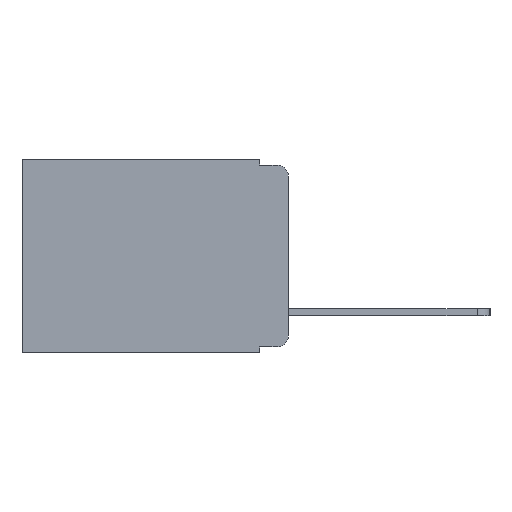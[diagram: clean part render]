
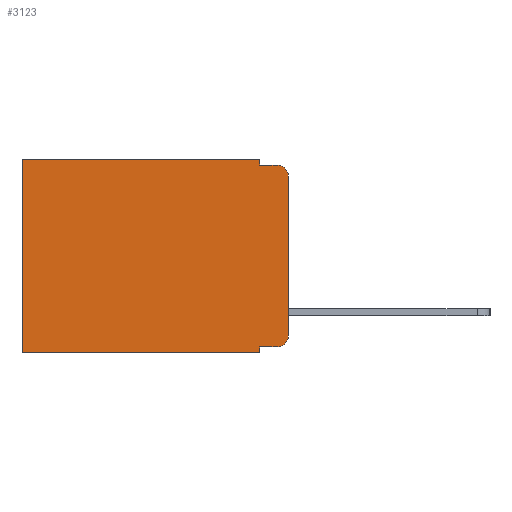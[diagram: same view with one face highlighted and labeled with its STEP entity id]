
A CAD part, left-side view. The second image highlights one B-rep face of the part: STEP entity #3123.
In plain terms, the highlighted planar face has unit normal (-1, 0, 0).
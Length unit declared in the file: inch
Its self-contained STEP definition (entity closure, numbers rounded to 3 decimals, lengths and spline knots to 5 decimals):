
#327 = ORIENTED_EDGE ( 'NONE', *, *, #18414, .F. ) ;
#622 = CARTESIAN_POINT ( 'NONE',  ( 0.298, 0., 0. ) ) ;
#1274 = CARTESIAN_POINT ( 'NONE',  ( 0.298, 0.473, 0. ) ) ;
#1833 = VERTEX_POINT ( 'NONE', #5368 ) ;
#2019 = ORIENTED_EDGE ( 'NONE', *, *, #11869, .T. ) ;
#2214 = VERTEX_POINT ( 'NONE', #1274 ) ;
#2249 = EDGE_CURVE ( 'NONE', #18084, #2214, #5671, .T. ) ;
#2390 = CARTESIAN_POINT ( 'NONE',  ( 0.298, 0.051, 0. ) ) ;
#2619 = VERTEX_POINT ( 'NONE', #6389 ) ;
#2701 = ORIENTED_EDGE ( 'NONE', *, *, #6005, .F. ) ;
#2780 = ORIENTED_EDGE ( 'NONE', *, *, #13232, .F. ) ;
#2804 = ORIENTED_EDGE ( 'NONE', *, *, #17581, .F. ) ;
#2856 = VERTEX_POINT ( 'NONE', #7756 ) ;
#2863 = DIRECTION ( 'NONE',  ( 0., 0., -1. ) ) ;
#2877 = CARTESIAN_POINT ( 'NONE',  ( 0.298, 0.051, -0.01 ) ) ;
#2908 = EDGE_CURVE ( 'NONE', #12253, #18066, #9824, .T. ) ;
#2993 = DIRECTION ( 'NONE',  ( 0., 0., -1. ) ) ;
#3123 = ADVANCED_FACE ( 'NONE', ( #16680 ), #18057, .F. ) ;
#3352 = VECTOR ( 'NONE', #12603, 39.37008 ) ;
#3385 = CARTESIAN_POINT ( 'NONE',  ( 0.298, 0., -0.313 ) ) ;
#3512 = CARTESIAN_POINT ( 'NONE',  ( 0.298, 0.02, -0.333 ) ) ;
#3734 = VECTOR ( 'NONE', #4436, 39.37008 ) ;
#3966 = DIRECTION ( 'NONE',  ( -1., 0., 0. ) ) ;
#3967 = DIRECTION ( 'NONE',  ( 0., 0., -1. ) ) ;
#4007 = CIRCLE ( 'NONE', #10460, 0.02 ) ;
#4109 = VERTEX_POINT ( 'NONE', #3385 ) ;
#4436 = DIRECTION ( 'NONE',  ( 0., -1., 0. ) ) ;
#4811 = CARTESIAN_POINT ( 'NONE',  ( 0.298, 0., -0.03 ) ) ;
#5027 = ORIENTED_EDGE ( 'NONE', *, *, #2908, .T. ) ;
#5180 = ORIENTED_EDGE ( 'NONE', *, *, #15065, .F. ) ;
#5368 = CARTESIAN_POINT ( 'NONE',  ( 0.298, 0.051, -0.01 ) ) ;
#5398 = CARTESIAN_POINT ( 'NONE',  ( 0.298, 0.051, 0. ) ) ;
#5437 = EDGE_CURVE ( 'NONE', #10813, #2856, #17249, .T. ) ;
#5496 = DIRECTION ( 'NONE',  ( -1., 0., 0. ) ) ;
#5534 = ORIENTED_EDGE ( 'NONE', *, *, #15301, .T. ) ;
#5671 = LINE ( 'NONE', #622, #16231 ) ;
#6005 = EDGE_CURVE ( 'NONE', #12253, #2619, #18819, .T. ) ;
#6211 = ORIENTED_EDGE ( 'NONE', *, *, #2249, .T. ) ;
#6229 = ORIENTED_EDGE ( 'NONE', *, *, #5437, .T. ) ;
#6389 = CARTESIAN_POINT ( 'NONE',  ( 0.298, 0.051, -0.343 ) ) ;
#6907 = CARTESIAN_POINT ( 'NONE',  ( 0.298, 0.473, -0.343 ) ) ;
#7387 = VECTOR ( 'NONE', #2993, 39.37008 ) ;
#7711 = DIRECTION ( 'NONE',  ( 0., -1., 0. ) ) ;
#7756 = CARTESIAN_POINT ( 'NONE',  ( 0.298, 0.02, -0.01 ) ) ;
#9770 = CARTESIAN_POINT ( 'NONE',  ( 0.298, 0., -0.343 ) ) ;
#9824 = LINE ( 'NONE', #15925, #13552 ) ;
#10341 = CARTESIAN_POINT ( 'NONE',  ( 0.298, 0.473, 0. ) ) ;
#10455 = VECTOR ( 'NONE', #3967, 39.37008 ) ;
#10460 = AXIS2_PLACEMENT_3D ( 'NONE', #12768, #3966, #14149 ) ;
#10813 = VERTEX_POINT ( 'NONE', #4811 ) ;
#10910 = LINE ( 'NONE', #2390, #10455 ) ;
#11118 = LINE ( 'NONE', #10341, #14409 ) ;
#11132 = DIRECTION ( 'NONE',  ( 0., 1., 0. ) ) ;
#11869 = EDGE_CURVE ( 'NONE', #18066, #4109, #4007, .T. ) ;
#12253 = VERTEX_POINT ( 'NONE', #14732 ) ;
#12603 = DIRECTION ( 'NONE',  ( 0., 1., 0. ) ) ;
#12768 = CARTESIAN_POINT ( 'NONE',  ( 0.298, 0.02, -0.313 ) ) ;
#13232 = EDGE_CURVE ( 'NONE', #1833, #2856, #19247, .T. ) ;
#13315 = AXIS2_PLACEMENT_3D ( 'NONE', #17642, #18265, #18280 ) ;
#13552 = VECTOR ( 'NONE', #7711, 39.37008 ) ;
#14128 = CARTESIAN_POINT ( 'NONE',  ( 0.298, 0.02, -0.03 ) ) ;
#14149 = DIRECTION ( 'NONE',  ( 0., 0., -1. ) ) ;
#14409 = VECTOR ( 'NONE', #2863, 39.37008 ) ;
#14444 = VERTEX_POINT ( 'NONE', #6907 ) ;
#14616 = CARTESIAN_POINT ( 'NONE',  ( 0.298, 0., 0. ) ) ;
#14732 = CARTESIAN_POINT ( 'NONE',  ( 0.298, 0.051, -0.333 ) ) ;
#14913 = LINE ( 'NONE', #14616, #7387 ) ;
#15065 = EDGE_CURVE ( 'NONE', #18084, #1833, #10910, .T. ) ;
#15242 = CARTESIAN_POINT ( 'NONE',  ( 0.298, 0.051, 0. ) ) ;
#15301 = EDGE_CURVE ( 'NONE', #2214, #14444, #11118, .T. ) ;
#15518 = DIRECTION ( 'NONE',  ( 0., 0., -1. ) ) ;
#15925 = CARTESIAN_POINT ( 'NONE',  ( 0.298, 0.051, -0.333 ) ) ;
#16231 = VECTOR ( 'NONE', #11132, 39.37008 ) ;
#16680 = FACE_OUTER_BOUND ( 'NONE', #18865, .T. ) ;
#17066 = AXIS2_PLACEMENT_3D ( 'NONE', #14128, #5496, #15518 ) ;
#17249 = CIRCLE ( 'NONE', #17066, 0.02 ) ;
#17581 = EDGE_CURVE ( 'NONE', #2619, #14444, #19080, .T. ) ;
#17642 = CARTESIAN_POINT ( 'NONE',  ( 0.298, 0., 0. ) ) ;
#18057 = PLANE ( 'NONE',  #13315 ) ;
#18066 = VERTEX_POINT ( 'NONE', #3512 ) ;
#18084 = VERTEX_POINT ( 'NONE', #15242 ) ;
#18265 = DIRECTION ( 'NONE',  ( 1., 0., 0. ) ) ;
#18280 = DIRECTION ( 'NONE',  ( 0., 0., -1. ) ) ;
#18361 = VECTOR ( 'NONE', #18437, 39.37008 ) ;
#18414 = EDGE_CURVE ( 'NONE', #10813, #4109, #14913, .T. ) ;
#18437 = DIRECTION ( 'NONE',  ( 0., 0., -1. ) ) ;
#18819 = LINE ( 'NONE', #5398, #18361 ) ;
#18865 = EDGE_LOOP ( 'NONE', ( #327, #6229, #2780, #5180, #6211, #5534, #2804, #2701, #5027, #2019 ) ) ;
#19080 = LINE ( 'NONE', #9770, #3352 ) ;
#19247 = LINE ( 'NONE', #2877, #3734 ) ;
